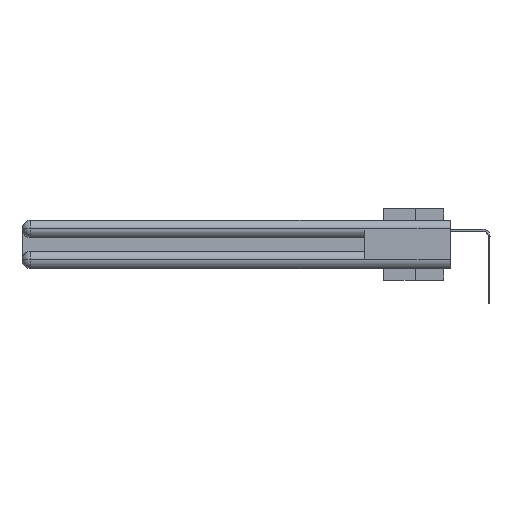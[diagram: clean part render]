
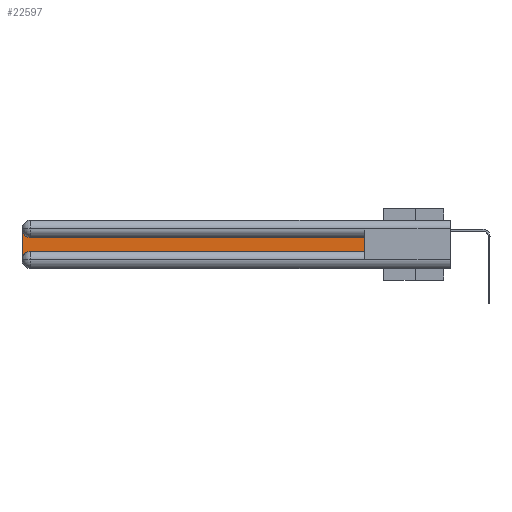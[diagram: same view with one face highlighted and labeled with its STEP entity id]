
A CAD part, left-side view. The second image highlights one B-rep face of the part: STEP entity #22597.
In plain terms, the highlighted planar face has unit normal (-1, 0, 0).
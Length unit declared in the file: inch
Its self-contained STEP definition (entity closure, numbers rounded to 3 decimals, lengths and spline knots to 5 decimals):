
#213 = ORIENTED_EDGE ( 'NONE', *, *, #8943, .T. ) ;
#758 = ORIENTED_EDGE ( 'NONE', *, *, #12304, .T. ) ;
#1368 = VERTEX_POINT ( 'NONE', #5131 ) ;
#1467 = EDGE_CURVE ( 'NONE', #11949, #33437, #7224, .T. ) ;
#2083 = PLANE ( 'NONE',  #8054 ) ;
#2403 = CARTESIAN_POINT ( 'NONE',  ( 0.075, 0.6, -0.2175 ) ) ;
#3592 = CARTESIAN_POINT ( 'NONE',  ( 0.075, 2.94, -0.0625 ) ) ;
#3666 = FACE_OUTER_BOUND ( 'NONE', #8935, .T. ) ;
#3747 = ORIENTED_EDGE ( 'NONE', *, *, #1467, .T. ) ;
#3779 = VECTOR ( 'NONE', #23078, 39.37008 ) ;
#5131 = CARTESIAN_POINT ( 'NONE',  ( 0.075, 2.94, -0.1225 ) ) ;
#5542 = ORIENTED_EDGE ( 'NONE', *, *, #16973, .T. ) ;
#7067 = CARTESIAN_POINT ( 'NONE',  ( 0.075, 3., -0.2175 ) ) ;
#7224 = CIRCLE ( 'NONE', #16469, 0.06 ) ;
#7587 = CARTESIAN_POINT ( 'NONE',  ( 0.075, 3., -0.1225 ) ) ;
#8054 = AXIS2_PLACEMENT_3D ( 'NONE', #7587, #33948, #25950 ) ;
#8434 = DIRECTION ( 'NONE',  ( 0., 0., -1. ) ) ;
#8935 = EDGE_LOOP ( 'NONE', ( #31195, #28721, #213, #3747, #758, #5542 ) ) ;
#8943 = EDGE_CURVE ( 'NONE', #27936, #11949, #23783, .T. ) ;
#9369 = CARTESIAN_POINT ( 'NONE',  ( 0.075, 0.6, -0.1225 ) ) ;
#10326 = DIRECTION ( 'NONE',  ( 0., 0., 1. ) ) ;
#11021 = CARTESIAN_POINT ( 'NONE',  ( 0.075, 3., -0.0625 ) ) ;
#11670 = LINE ( 'NONE', #2403, #27496 ) ;
#11949 = VERTEX_POINT ( 'NONE', #14225 ) ;
#12304 = EDGE_CURVE ( 'NONE', #33437, #21887, #23705, .T. ) ;
#12887 = CARTESIAN_POINT ( 'NONE',  ( 0.075, 2.94, -0.2175 ) ) ;
#14225 = CARTESIAN_POINT ( 'NONE',  ( 0.075, 3., -0.2775 ) ) ;
#14561 = DIRECTION ( 'NONE',  ( 1., 0., 0. ) ) ;
#14608 = DIRECTION ( 'NONE',  ( 0., 0., -1. ) ) ;
#16469 = AXIS2_PLACEMENT_3D ( 'NONE', #21577, #24255, #8434 ) ;
#16767 = VERTEX_POINT ( 'NONE', #17310 ) ;
#16973 = EDGE_CURVE ( 'NONE', #21887, #16767, #11670, .T. ) ;
#16988 = DIRECTION ( 'NONE',  ( 0., 0., -1. ) ) ;
#17310 = CARTESIAN_POINT ( 'NONE',  ( 0.075, 0.6, -0.1225 ) ) ;
#19284 = VECTOR ( 'NONE', #30961, 39.37008 ) ;
#21577 = CARTESIAN_POINT ( 'NONE',  ( 0.075, 2.94, -0.2775 ) ) ;
#21804 = LINE ( 'NONE', #9369, #19284 ) ;
#21887 = VERTEX_POINT ( 'NONE', #33640 ) ;
#22597 = ADVANCED_FACE ( 'NONE', ( #3666 ), #2083, .F. ) ;
#23078 = DIRECTION ( 'NONE',  ( 0., -1., 0. ) ) ;
#23705 = LINE ( 'NONE', #33603, #3779 ) ;
#23783 = LINE ( 'NONE', #7067, #29977 ) ;
#24255 = DIRECTION ( 'NONE',  ( 1., 0., 0. ) ) ;
#24521 = EDGE_CURVE ( 'NONE', #1368, #27936, #26383, .T. ) ;
#25465 = AXIS2_PLACEMENT_3D ( 'NONE', #3592, #14561, #16988 ) ;
#25950 = DIRECTION ( 'NONE',  ( 0., 0., -1. ) ) ;
#26383 = CIRCLE ( 'NONE', #25465, 0.06 ) ;
#26968 = EDGE_CURVE ( 'NONE', #16767, #1368, #21804, .T. ) ;
#27496 = VECTOR ( 'NONE', #10326, 39.37008 ) ;
#27936 = VERTEX_POINT ( 'NONE', #11021 ) ;
#28721 = ORIENTED_EDGE ( 'NONE', *, *, #24521, .T. ) ;
#29977 = VECTOR ( 'NONE', #14608, 39.37008 ) ;
#30961 = DIRECTION ( 'NONE',  ( 0., 1., 0. ) ) ;
#31195 = ORIENTED_EDGE ( 'NONE', *, *, #26968, .T. ) ;
#33437 = VERTEX_POINT ( 'NONE', #12887 ) ;
#33603 = CARTESIAN_POINT ( 'NONE',  ( 0.075, 0.6, -0.2175 ) ) ;
#33640 = CARTESIAN_POINT ( 'NONE',  ( 0.075, 0.6, -0.2175 ) ) ;
#33948 = DIRECTION ( 'NONE',  ( 1., 0., 0. ) ) ;
